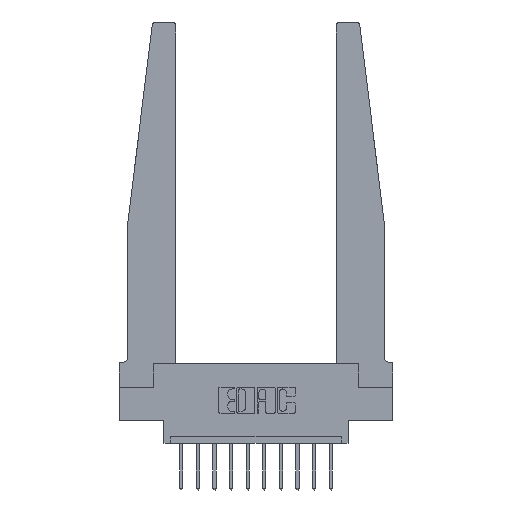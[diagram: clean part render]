
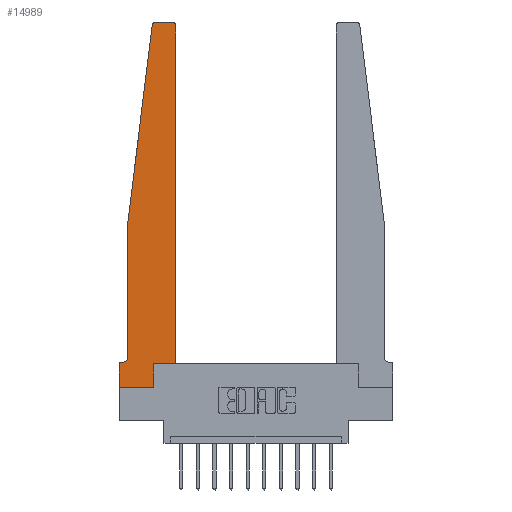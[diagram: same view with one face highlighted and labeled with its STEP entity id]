
A CAD part, top view. The second image highlights one B-rep face of the part: STEP entity #14989.
In plain terms, the highlighted planar face has unit normal (0, 0, 1).
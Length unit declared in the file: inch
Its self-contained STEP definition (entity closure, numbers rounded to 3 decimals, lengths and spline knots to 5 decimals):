
#933 = DIRECTION ( 'NONE',  ( -1., 0., 0. ) ) ;
#962 = CARTESIAN_POINT ( 'NONE',  ( 0.2605, 0., 0.37 ) ) ;
#1247 = ORIENTED_EDGE ( 'NONE', *, *, #11894, .T. ) ;
#1563 = VERTEX_POINT ( 'NONE', #1991 ) ;
#1569 = VERTEX_POINT ( 'NONE', #11222 ) ;
#1746 = DIRECTION ( 'NONE',  ( 0., -1., 0. ) ) ;
#1991 = CARTESIAN_POINT ( 'NONE',  ( 0.065, 1.25, 0.37 ) ) ;
#2183 = LINE ( 'NONE', #7143, #10238 ) ;
#2252 = DIRECTION ( 'NONE',  ( 0., 0., 1. ) ) ;
#3019 = CARTESIAN_POINT ( 'NONE',  ( 0., 0., 0.37 ) ) ;
#3234 = DIRECTION ( 'NONE',  ( 0., -1., 0. ) ) ;
#3291 = CARTESIAN_POINT ( 'NONE',  ( 0.065, 0.2375, 0.37 ) ) ;
#3306 = AXIS2_PLACEMENT_3D ( 'NONE', #5817, #10690, #15670 ) ;
#3651 = VECTOR ( 'NONE', #6036, 39.37008 ) ;
#3740 = CARTESIAN_POINT ( 'NONE',  ( 0.425, 2.72, 0.37 ) ) ;
#3741 = CARTESIAN_POINT ( 'NONE',  ( 0.065, 1.25, 0.37 ) ) ;
#4123 = ORIENTED_EDGE ( 'NONE', *, *, #14356, .T. ) ;
#4224 = VECTOR ( 'NONE', #3234, 39.37008 ) ;
#4283 = CIRCLE ( 'NONE', #13278, 0.03 ) ;
#4352 = DIRECTION ( 'NONE',  ( 0., 1., 0. ) ) ;
#4360 = CARTESIAN_POINT ( 'NONE',  ( 0., 0., 0.37 ) ) ;
#4434 = VERTEX_POINT ( 'NONE', #3740 ) ;
#4686 = EDGE_CURVE ( 'NONE', #15337, #8688, #5760, .T. ) ;
#4715 = DIRECTION ( 'NONE',  ( 0., 1., 0. ) ) ;
#5135 = EDGE_CURVE ( 'NONE', #1569, #6362, #9797, .T. ) ;
#5240 = CARTESIAN_POINT ( 'NONE',  ( 0., 0., 0.37 ) ) ;
#5574 = LINE ( 'NONE', #14084, #8262 ) ;
#5637 = ORIENTED_EDGE ( 'NONE', *, *, #7886, .T. ) ;
#5760 = LINE ( 'NONE', #7038, #14948 ) ;
#5817 = CARTESIAN_POINT ( 'NONE',  ( 0.015, 0.2375, 0.37 ) ) ;
#5831 = VERTEX_POINT ( 'NONE', #962 ) ;
#6036 = DIRECTION ( 'NONE',  ( 1., 0., 0. ) ) ;
#6070 = ORIENTED_EDGE ( 'NONE', *, *, #11315, .T. ) ;
#6094 = VERTEX_POINT ( 'NONE', #10459 ) ;
#6362 = VERTEX_POINT ( 'NONE', #7575 ) ;
#6628 = LINE ( 'NONE', #4360, #11949 ) ;
#6679 = EDGE_LOOP ( 'NONE', ( #15547, #11491, #11943, #5637, #10175, #11033, #11859, #6070, #4123, #14351, #15213, #1247 ) ) ;
#6729 = FACE_OUTER_BOUND ( 'NONE', #6679, .T. ) ;
#7038 = CARTESIAN_POINT ( 'NONE',  ( 0.25, 2.75, 0.37 ) ) ;
#7143 = CARTESIAN_POINT ( 'NONE',  ( 0.425, 0.18, 0.37 ) ) ;
#7284 = EDGE_CURVE ( 'NONE', #11247, #10140, #6628, .T. ) ;
#7448 = VECTOR ( 'NONE', #4352, 39.37008 ) ;
#7575 = CARTESIAN_POINT ( 'NONE',  ( 0.425, 0.18, 0.37 ) ) ;
#7858 = DIRECTION ( 'NONE',  ( 1., 0., 0. ) ) ;
#7886 = EDGE_CURVE ( 'NONE', #1563, #14681, #14471, .T. ) ;
#7926 = DIRECTION ( 'NONE',  ( 1., 0., 0. ) ) ;
#8249 = EDGE_CURVE ( 'NONE', #10306, #1563, #9849, .T. ) ;
#8262 = VECTOR ( 'NONE', #933, 39.37008 ) ;
#8303 = CARTESIAN_POINT ( 'NONE',  ( 0.065, 1.25, 0.37 ) ) ;
#8688 = VERTEX_POINT ( 'NONE', #9242 ) ;
#8889 = CARTESIAN_POINT ( 'NONE',  ( 0., 0.1875, 0.37 ) ) ;
#9242 = CARTESIAN_POINT ( 'NONE',  ( 0.27653, 2.75, 0.37 ) ) ;
#9790 = AXIS2_PLACEMENT_3D ( 'NONE', #8889, #11371, #7858 ) ;
#9797 = LINE ( 'NONE', #13347, #3651 ) ;
#9849 = LINE ( 'NONE', #3741, #14510 ) ;
#10076 = PLANE ( 'NONE',  #9790 ) ;
#10140 = VERTEX_POINT ( 'NONE', #5240 ) ;
#10175 = ORIENTED_EDGE ( 'NONE', *, *, #12540, .T. ) ;
#10238 = VECTOR ( 'NONE', #4715, 39.37008 ) ;
#10306 = VERTEX_POINT ( 'NONE', #12005 ) ;
#10459 = CARTESIAN_POINT ( 'NONE',  ( 0.015, 0.1875, 0.37 ) ) ;
#10475 = CIRCLE ( 'NONE', #12557, 0.03 ) ;
#10690 = DIRECTION ( 'NONE',  ( 0., 0., -1. ) ) ;
#10832 = DIRECTION ( 'NONE',  ( 0., 0., 1. ) ) ;
#10836 = LINE ( 'NONE', #12146, #7448 ) ;
#10973 = DIRECTION ( 'NONE',  ( -0.122, -0.992, 0. ) ) ;
#11033 = ORIENTED_EDGE ( 'NONE', *, *, #15380, .T. ) ;
#11222 = CARTESIAN_POINT ( 'NONE',  ( 0.2605, 0.18, 0.37 ) ) ;
#11247 = VERTEX_POINT ( 'NONE', #14170 ) ;
#11315 = EDGE_CURVE ( 'NONE', #10140, #5831, #14015, .T. ) ;
#11371 = DIRECTION ( 'NONE',  ( 0., 0., 1. ) ) ;
#11491 = ORIENTED_EDGE ( 'NONE', *, *, #13601, .T. ) ;
#11495 = CIRCLE ( 'NONE', #3306, 0.05 ) ;
#11859 = ORIENTED_EDGE ( 'NONE', *, *, #7284, .T. ) ;
#11894 = EDGE_CURVE ( 'NONE', #4434, #15337, #4283, .T. ) ;
#11943 = ORIENTED_EDGE ( 'NONE', *, *, #8249, .T. ) ;
#11949 = VECTOR ( 'NONE', #1746, 39.37008 ) ;
#12005 = CARTESIAN_POINT ( 'NONE',  ( 0.24675, 2.72367, 0.37 ) ) ;
#12146 = CARTESIAN_POINT ( 'NONE',  ( 0.2605, 0.18, 0.37 ) ) ;
#12540 = EDGE_CURVE ( 'NONE', #14681, #6094, #11495, .T. ) ;
#12557 = AXIS2_PLACEMENT_3D ( 'NONE', #13084, #2252, #15639 ) ;
#13067 = DIRECTION ( 'NONE',  ( -1., 0., 0. ) ) ;
#13084 = CARTESIAN_POINT ( 'NONE',  ( 0.27653, 2.72, 0.37 ) ) ;
#13266 = VECTOR ( 'NONE', #7926, 39.37008 ) ;
#13278 = AXIS2_PLACEMENT_3D ( 'NONE', #15732, #10832, #14532 ) ;
#13347 = CARTESIAN_POINT ( 'NONE',  ( 0.425, 0.18, 0.37 ) ) ;
#13601 = EDGE_CURVE ( 'NONE', #8688, #10306, #10475, .T. ) ;
#14015 = LINE ( 'NONE', #3019, #13266 ) ;
#14084 = CARTESIAN_POINT ( 'NONE',  ( 0.065, 0.1875, 0.37 ) ) ;
#14170 = CARTESIAN_POINT ( 'NONE',  ( 0., 0.1875, 0.37 ) ) ;
#14351 = ORIENTED_EDGE ( 'NONE', *, *, #5135, .T. ) ;
#14356 = EDGE_CURVE ( 'NONE', #5831, #1569, #10836, .T. ) ;
#14471 = LINE ( 'NONE', #8303, #4224 ) ;
#14510 = VECTOR ( 'NONE', #10973, 39.37008 ) ;
#14532 = DIRECTION ( 'NONE',  ( 1., 0., 0. ) ) ;
#14681 = VERTEX_POINT ( 'NONE', #3291 ) ;
#14742 = EDGE_CURVE ( 'NONE', #6362, #4434, #2183, .T. ) ;
#14948 = VECTOR ( 'NONE', #13067, 39.37008 ) ;
#14989 = ADVANCED_FACE ( 'NONE', ( #6729 ), #10076, .T. ) ;
#15118 = CARTESIAN_POINT ( 'NONE',  ( 0.395, 2.75, 0.37 ) ) ;
#15213 = ORIENTED_EDGE ( 'NONE', *, *, #14742, .T. ) ;
#15337 = VERTEX_POINT ( 'NONE', #15118 ) ;
#15380 = EDGE_CURVE ( 'NONE', #6094, #11247, #5574, .T. ) ;
#15547 = ORIENTED_EDGE ( 'NONE', *, *, #4686, .T. ) ;
#15639 = DIRECTION ( 'NONE',  ( 1., 0., 0. ) ) ;
#15670 = DIRECTION ( 'NONE',  ( -1., 0., 0. ) ) ;
#15732 = CARTESIAN_POINT ( 'NONE',  ( 0.395, 2.72, 0.37 ) ) ;
